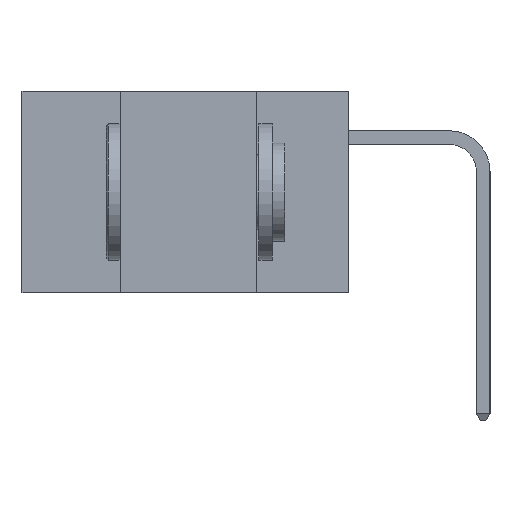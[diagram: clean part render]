
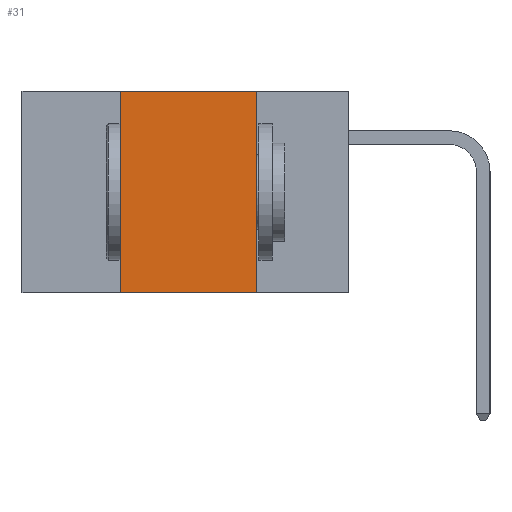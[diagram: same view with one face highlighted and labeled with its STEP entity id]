
A CAD part, left-side view. The second image highlights one B-rep face of the part: STEP entity #31.
In plain terms, the highlighted planar face has unit normal (-1, 0, 0).
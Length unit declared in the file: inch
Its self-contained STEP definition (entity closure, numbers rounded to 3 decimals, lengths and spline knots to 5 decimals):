
#31 = ADVANCED_FACE ( 'NONE', ( #7360 ), #8414, .F. ) ;
#71 = AXIS2_PLACEMENT_3D ( 'NONE', #8480, #6157, #8429 ) ;
#462 = DIRECTION ( 'NONE',  ( 0., -1., 0. ) ) ;
#944 = LINE ( 'NONE', #5851, #5432 ) ;
#1017 = EDGE_CURVE ( 'NONE', #8302, #7131, #944, .T. ) ;
#3018 = ORIENTED_EDGE ( 'NONE', *, *, #1017, .F. ) ;
#3337 = VECTOR ( 'NONE', #462, 39.37008 ) ;
#3465 = VERTEX_POINT ( 'NONE', #9172 ) ;
#4051 = EDGE_CURVE ( 'NONE', #4238, #7131, #4574, .T. ) ;
#4154 = CARTESIAN_POINT ( 'NONE',  ( 0., 0.17, -0.37 ) ) ;
#4238 = VERTEX_POINT ( 'NONE', #9728 ) ;
#4341 = LINE ( 'NONE', #9353, #6168 ) ;
#4574 = LINE ( 'NONE', #7496, #6367 ) ;
#4722 = ORIENTED_EDGE ( 'NONE', *, *, #9201, .F. ) ;
#4898 = DIRECTION ( 'NONE',  ( 0., 0., -1. ) ) ;
#5207 = LINE ( 'NONE', #5545, #3337 ) ;
#5432 = VECTOR ( 'NONE', #4898, 39.37008 ) ;
#5545 = CARTESIAN_POINT ( 'NONE',  ( 0., 0.6, 0. ) ) ;
#5623 = EDGE_LOOP ( 'NONE', ( #3018, #4722, #6060, #7058 ) ) ;
#5690 = DIRECTION ( 'NONE',  ( 0., 0., 1. ) ) ;
#5851 = CARTESIAN_POINT ( 'NONE',  ( 0., 0.17, 0. ) ) ;
#6060 = ORIENTED_EDGE ( 'NONE', *, *, #8576, .F. ) ;
#6157 = DIRECTION ( 'NONE',  ( 1., 0., 0. ) ) ;
#6168 = VECTOR ( 'NONE', #5690, 39.37008 ) ;
#6367 = VECTOR ( 'NONE', #7919, 39.37008 ) ;
#7058 = ORIENTED_EDGE ( 'NONE', *, *, #4051, .T. ) ;
#7131 = VERTEX_POINT ( 'NONE', #4154 ) ;
#7360 = FACE_OUTER_BOUND ( 'NONE', #5623, .T. ) ;
#7496 = CARTESIAN_POINT ( 'NONE',  ( 0., 0.6, -0.37 ) ) ;
#7919 = DIRECTION ( 'NONE',  ( 0., -1., 0. ) ) ;
#8302 = VERTEX_POINT ( 'NONE', #8440 ) ;
#8414 = PLANE ( 'NONE',  #71 ) ;
#8429 = DIRECTION ( 'NONE',  ( 0., 0., -1. ) ) ;
#8440 = CARTESIAN_POINT ( 'NONE',  ( 0., 0.17, 0. ) ) ;
#8480 = CARTESIAN_POINT ( 'NONE',  ( 0., 0.6, 0. ) ) ;
#8576 = EDGE_CURVE ( 'NONE', #4238, #3465, #4341, .T. ) ;
#9172 = CARTESIAN_POINT ( 'NONE',  ( 0., 0.42, 0. ) ) ;
#9201 = EDGE_CURVE ( 'NONE', #3465, #8302, #5207, .T. ) ;
#9353 = CARTESIAN_POINT ( 'NONE',  ( 0., 0.42, 0. ) ) ;
#9728 = CARTESIAN_POINT ( 'NONE',  ( 0., 0.42, -0.37 ) ) ;
